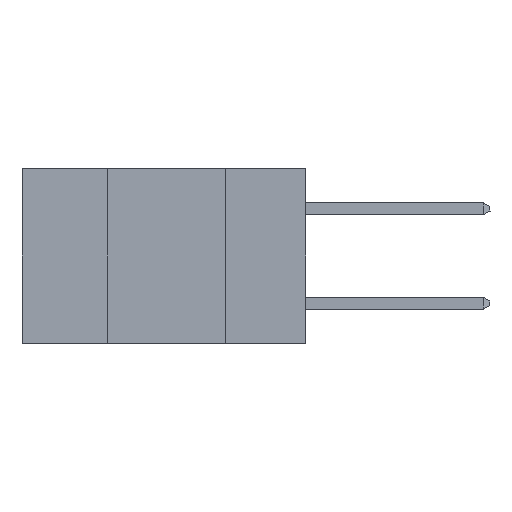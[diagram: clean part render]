
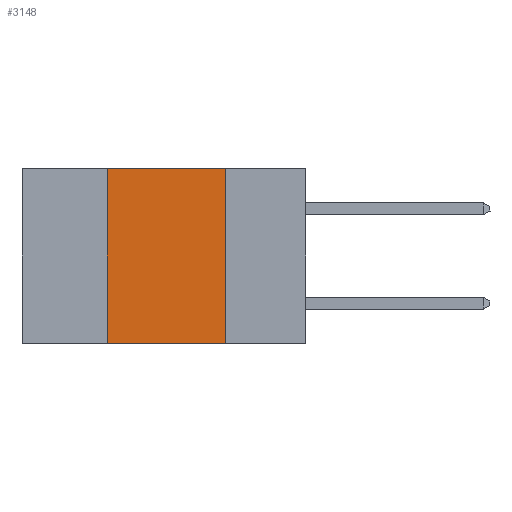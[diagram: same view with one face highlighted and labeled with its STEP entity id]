
A CAD part, left-side view. The second image highlights one B-rep face of the part: STEP entity #3148.
In plain terms, the highlighted planar face has unit normal (-1, 0, 0).
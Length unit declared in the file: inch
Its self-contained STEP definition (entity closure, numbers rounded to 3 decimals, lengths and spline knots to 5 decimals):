
#371 = EDGE_LOOP ( 'NONE', ( #5427, #4391, #4168, #1083 ) ) ;
#573 = EDGE_CURVE ( 'NONE', #7230, #4271, #9276, .T. ) ;
#588 = LINE ( 'NONE', #1312, #7447 ) ;
#1083 = ORIENTED_EDGE ( 'NONE', *, *, #573, .T. ) ;
#1177 = CARTESIAN_POINT ( 'NONE',  ( 0., 0.42, 0. ) ) ;
#1312 = CARTESIAN_POINT ( 'NONE',  ( 0., 0.6, 0. ) ) ;
#1748 = LINE ( 'NONE', #1177, #4841 ) ;
#1925 = VERTEX_POINT ( 'NONE', #5088 ) ;
#1934 = LINE ( 'NONE', #7174, #9048 ) ;
#2783 = CARTESIAN_POINT ( 'NONE',  ( 0., 0.42, -0.37 ) ) ;
#3031 = PLANE ( 'NONE',  #8679 ) ;
#3148 = ADVANCED_FACE ( 'NONE', ( #3165 ), #3031, .F. ) ;
#3165 = FACE_OUTER_BOUND ( 'NONE', #371, .T. ) ;
#4168 = ORIENTED_EDGE ( 'NONE', *, *, #5360, .F. ) ;
#4271 = VERTEX_POINT ( 'NONE', #4316 ) ;
#4316 = CARTESIAN_POINT ( 'NONE',  ( 0., 0.17, -0.37 ) ) ;
#4391 = ORIENTED_EDGE ( 'NONE', *, *, #6174, .F. ) ;
#4841 = VECTOR ( 'NONE', #7727, 39.37008 ) ;
#5088 = CARTESIAN_POINT ( 'NONE',  ( 0., 0.42, 0. ) ) ;
#5288 = CARTESIAN_POINT ( 'NONE',  ( 0., 0.6, 0. ) ) ;
#5307 = CARTESIAN_POINT ( 'NONE',  ( 0., 0.17, 0. ) ) ;
#5360 = EDGE_CURVE ( 'NONE', #7230, #1925, #1748, .T. ) ;
#5427 = ORIENTED_EDGE ( 'NONE', *, *, #7642, .F. ) ;
#5869 = VERTEX_POINT ( 'NONE', #5307 ) ;
#6174 = EDGE_CURVE ( 'NONE', #1925, #5869, #588, .T. ) ;
#6434 = VECTOR ( 'NONE', #6446, 39.37008 ) ;
#6446 = DIRECTION ( 'NONE',  ( 0., -1., 0. ) ) ;
#7150 = DIRECTION ( 'NONE',  ( 0., -1., 0. ) ) ;
#7158 = CARTESIAN_POINT ( 'NONE',  ( 0., 0.6, -0.37 ) ) ;
#7174 = CARTESIAN_POINT ( 'NONE',  ( 0., 0.17, 0. ) ) ;
#7230 = VERTEX_POINT ( 'NONE', #2783 ) ;
#7447 = VECTOR ( 'NONE', #7150, 39.37008 ) ;
#7642 = EDGE_CURVE ( 'NONE', #5869, #4271, #1934, .T. ) ;
#7727 = DIRECTION ( 'NONE',  ( 0., 0., 1. ) ) ;
#7906 = DIRECTION ( 'NONE',  ( 0., 0., -1. ) ) ;
#8158 = DIRECTION ( 'NONE',  ( 1., 0., 0. ) ) ;
#8679 = AXIS2_PLACEMENT_3D ( 'NONE', #5288, #8158, #8893 ) ;
#8893 = DIRECTION ( 'NONE',  ( 0., 0., -1. ) ) ;
#9048 = VECTOR ( 'NONE', #7906, 39.37008 ) ;
#9276 = LINE ( 'NONE', #7158, #6434 ) ;
